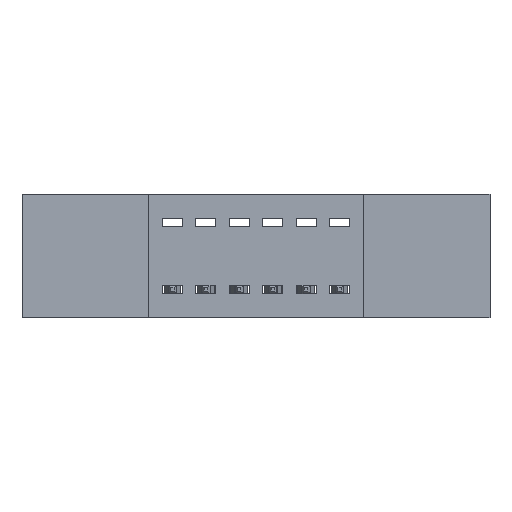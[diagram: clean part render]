
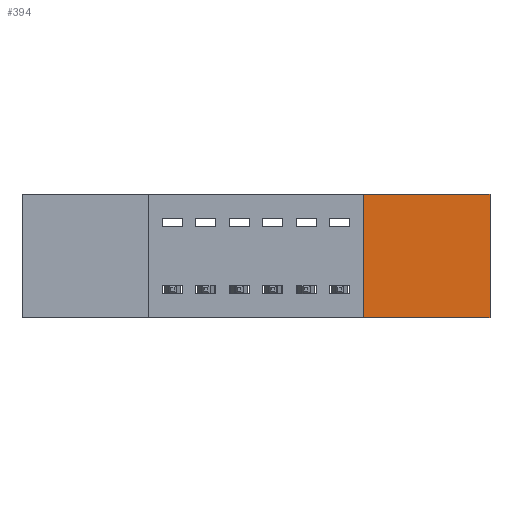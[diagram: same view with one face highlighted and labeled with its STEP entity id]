
A CAD part, front view. The second image highlights one B-rep face of the part: STEP entity #394.
In plain terms, the highlighted planar face has unit normal (0, -1, 0).
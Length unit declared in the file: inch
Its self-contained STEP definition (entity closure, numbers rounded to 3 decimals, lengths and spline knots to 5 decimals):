
#74 = CARTESIAN_POINT ( 'NONE',  ( 1.023, 0., 0. ) ) ;
#289 = CARTESIAN_POINT ( 'NONE',  ( 1.4, 0., 0. ) ) ;
#394 = ADVANCED_FACE ( 'NONE', ( #1617 ), #5612, .T. ) ;
#500 = VERTEX_POINT ( 'NONE', #4753 ) ;
#579 = VECTOR ( 'NONE', #2221, 39.37008 ) ;
#793 = CARTESIAN_POINT ( 'NONE',  ( 0., 0., -0.37 ) ) ;
#924 = VERTEX_POINT ( 'NONE', #74 ) ;
#1142 = CARTESIAN_POINT ( 'NONE',  ( 1.4, 0., 0. ) ) ;
#1280 = DIRECTION ( 'NONE',  ( 0., 0., -1. ) ) ;
#1451 = VERTEX_POINT ( 'NONE', #4017 ) ;
#1617 = FACE_OUTER_BOUND ( 'NONE', #1686, .T. ) ;
#1686 = EDGE_LOOP ( 'NONE', ( #5844, #2514, #7501, #6561 ) ) ;
#2221 = DIRECTION ( 'NONE',  ( -1., 0., 0. ) ) ;
#2250 = VECTOR ( 'NONE', #3688, 39.37008 ) ;
#2480 = VERTEX_POINT ( 'NONE', #1142 ) ;
#2514 = ORIENTED_EDGE ( 'NONE', *, *, #7894, .F. ) ;
#3115 = CARTESIAN_POINT ( 'NONE',  ( 0., 0., 0. ) ) ;
#3295 = EDGE_CURVE ( 'NONE', #1451, #924, #6962, .T. ) ;
#3314 = VECTOR ( 'NONE', #4702, 39.37008 ) ;
#3341 = CARTESIAN_POINT ( 'NONE',  ( 0., 0., -0.37 ) ) ;
#3688 = DIRECTION ( 'NONE',  ( 1., 0., 0. ) ) ;
#4017 = CARTESIAN_POINT ( 'NONE',  ( 1.023, 0., -0.37 ) ) ;
#4282 = DIRECTION ( 'NONE',  ( 0., 0., -1. ) ) ;
#4702 = DIRECTION ( 'NONE',  ( 0., 0., 1. ) ) ;
#4753 = CARTESIAN_POINT ( 'NONE',  ( 1.4, 0., -0.37 ) ) ;
#5053 = VECTOR ( 'NONE', #4282, 39.37008 ) ;
#5412 = LINE ( 'NONE', #3115, #2250 ) ;
#5612 = PLANE ( 'NONE',  #6672 ) ;
#5701 = CARTESIAN_POINT ( 'NONE',  ( 1.023, 0., -0.37 ) ) ;
#5771 = EDGE_CURVE ( 'NONE', #2480, #500, #6619, .T. ) ;
#5844 = ORIENTED_EDGE ( 'NONE', *, *, #3295, .F. ) ;
#5856 = DIRECTION ( 'NONE',  ( 0., -1., 0. ) ) ;
#6380 = EDGE_CURVE ( 'NONE', #924, #2480, #5412, .T. ) ;
#6561 = ORIENTED_EDGE ( 'NONE', *, *, #6380, .F. ) ;
#6619 = LINE ( 'NONE', #289, #5053 ) ;
#6672 = AXIS2_PLACEMENT_3D ( 'NONE', #793, #5856, #1280 ) ;
#6962 = LINE ( 'NONE', #5701, #3314 ) ;
#6985 = LINE ( 'NONE', #3341, #579 ) ;
#7501 = ORIENTED_EDGE ( 'NONE', *, *, #5771, .F. ) ;
#7894 = EDGE_CURVE ( 'NONE', #500, #1451, #6985, .T. ) ;
